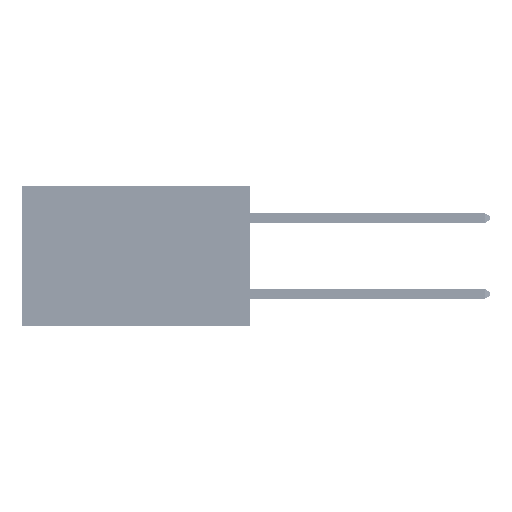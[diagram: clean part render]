
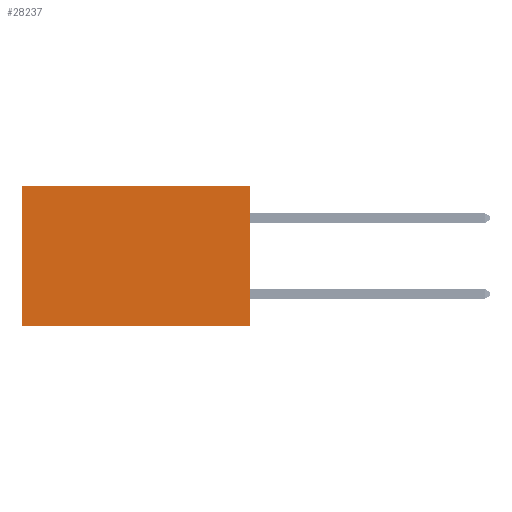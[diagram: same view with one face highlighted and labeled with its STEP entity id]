
A CAD part, left-side view. The second image highlights one B-rep face of the part: STEP entity #28237.
In plain terms, the highlighted planar face has unit normal (-1, 0, 0).
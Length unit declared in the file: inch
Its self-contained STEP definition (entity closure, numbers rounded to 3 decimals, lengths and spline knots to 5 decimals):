
#1443 = LINE ( 'NONE', #42614, #3135 ) ;
#3135 = VECTOR ( 'NONE', #35083, 39.37008 ) ;
#4101 = CARTESIAN_POINT ( 'NONE',  ( 0.2875, 0.6, 0. ) ) ;
#6608 = PLANE ( 'NONE',  #46578 ) ;
#8476 = CARTESIAN_POINT ( 'NONE',  ( 0.2875, 0., 0. ) ) ;
#10167 = CARTESIAN_POINT ( 'NONE',  ( 0.2875, 0., 0. ) ) ;
#11372 = EDGE_LOOP ( 'NONE', ( #20215, #17932, #21474, #33434 ) ) ;
#11390 = CARTESIAN_POINT ( 'NONE',  ( 0.2875, 0., 0. ) ) ;
#11609 = CARTESIAN_POINT ( 'NONE',  ( 0.2875, 0.6, -0.37 ) ) ;
#14446 = LINE ( 'NONE', #32028, #21921 ) ;
#17932 = ORIENTED_EDGE ( 'NONE', *, *, #41153, .F. ) ;
#18050 = CARTESIAN_POINT ( 'NONE',  ( 0.2875, 0.6, 0. ) ) ;
#19303 = VERTEX_POINT ( 'NONE', #18050 ) ;
#20215 = ORIENTED_EDGE ( 'NONE', *, *, #38191, .T. ) ;
#20803 = DIRECTION ( 'NONE',  ( 0., 0., -1. ) ) ;
#21474 = ORIENTED_EDGE ( 'NONE', *, *, #37859, .F. ) ;
#21921 = VECTOR ( 'NONE', #39573, 39.37008 ) ;
#22989 = DIRECTION ( 'NONE',  ( 0., 1., 0. ) ) ;
#25019 = EDGE_CURVE ( 'NONE', #41970, #19303, #38578, .T. ) ;
#25377 = LINE ( 'NONE', #4101, #46667 ) ;
#28237 = ADVANCED_FACE ( 'NONE', ( #36495 ), #6608, .F. ) ;
#29918 = DIRECTION ( 'NONE',  ( 0., 0., -1. ) ) ;
#32028 = CARTESIAN_POINT ( 'NONE',  ( 0.2875, 0., 0. ) ) ;
#33434 = ORIENTED_EDGE ( 'NONE', *, *, #25019, .T. ) ;
#33524 = VERTEX_POINT ( 'NONE', #11609 ) ;
#33793 = VERTEX_POINT ( 'NONE', #45576 ) ;
#35083 = DIRECTION ( 'NONE',  ( 0., 1., 0. ) ) ;
#35931 = DIRECTION ( 'NONE',  ( 1., 0., 0. ) ) ;
#36495 = FACE_OUTER_BOUND ( 'NONE', #11372, .T. ) ;
#37859 = EDGE_CURVE ( 'NONE', #41970, #33793, #14446, .T. ) ;
#38191 = EDGE_CURVE ( 'NONE', #19303, #33524, #25377, .T. ) ;
#38578 = LINE ( 'NONE', #8476, #43731 ) ;
#39573 = DIRECTION ( 'NONE',  ( 0., 0., -1. ) ) ;
#41153 = EDGE_CURVE ( 'NONE', #33793, #33524, #1443, .T. ) ;
#41970 = VERTEX_POINT ( 'NONE', #11390 ) ;
#42614 = CARTESIAN_POINT ( 'NONE',  ( 0.2875, 0., -0.37 ) ) ;
#43731 = VECTOR ( 'NONE', #22989, 39.37008 ) ;
#45576 = CARTESIAN_POINT ( 'NONE',  ( 0.2875, 0., -0.37 ) ) ;
#46578 = AXIS2_PLACEMENT_3D ( 'NONE', #10167, #35931, #20803 ) ;
#46667 = VECTOR ( 'NONE', #29918, 39.37008 ) ;
